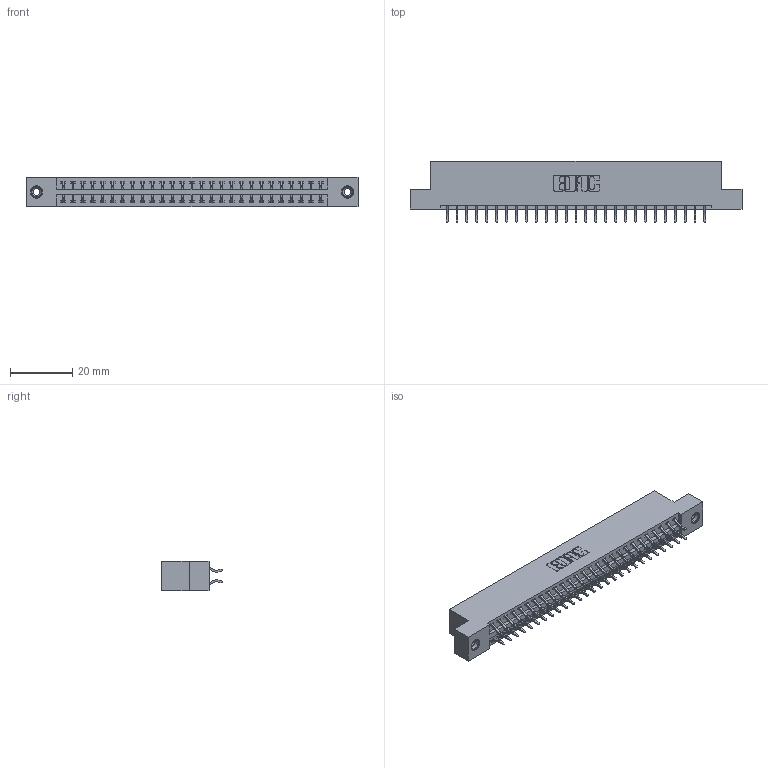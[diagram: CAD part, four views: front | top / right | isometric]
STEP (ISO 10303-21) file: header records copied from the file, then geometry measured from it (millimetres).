
FILE_DESCRIPTION (( 'STEP AP203' ), '1' );
FILE_NAME ('346-054-556-208.STEP', '2022-05-21T04:01:39', ( '' ), ( '' ), 'SwSTEP 2.0', 'SolidWorks 2020', '' );
FILE_SCHEMA (( 'CONFIG_CONTROL_DESIGN' ));
Length unit declared in the file: inch
Products named in the file (4): 346 Part_Flush Mounting Lugs - 0.156 Dia-TI; 345-292-001_556 Tail; 346-054-556-208; 345-250-001_345-250-003-102
Assembly tree (57 placements, depth 2):
  346-054-556-208
    346 Part_Flush Mounting Lugs - 0.156 Dia-TI
    345-292-001_556 Tail  x54
    345-250-001_345-250-003-102  x2
Bounding box: 106.3 x 19.57 x 9.4 mm (x, y, z)
Volume: 10240.3 mm3; surface area: 13810.1 mm2
Topology: 57 solids, 57 shells, 3314 faces, 9807 edges, 6458 vertices
Faces by surface type: plane 2214, cylinder 1084, cone 12, torus 4
Entity records: 21046 total; most frequent: CARTESIAN_POINT 3487, ORIENTED_EDGE 3402, DIRECTION 3139, EDGE_CURVE 1701, LINE 1433, VECTOR 1433, VERTEX_POINT 1128, AXIS2_PLACEMENT_3D 853
